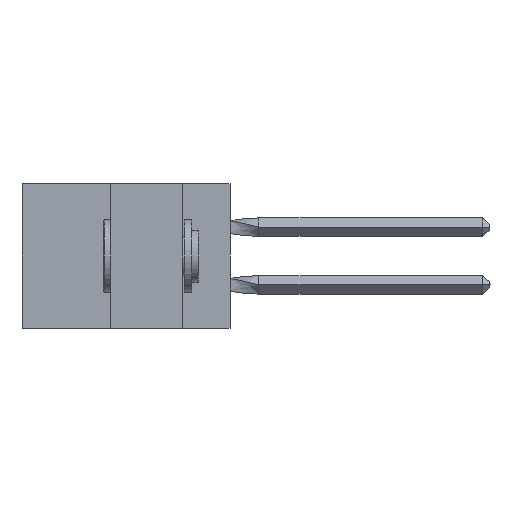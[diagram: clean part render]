
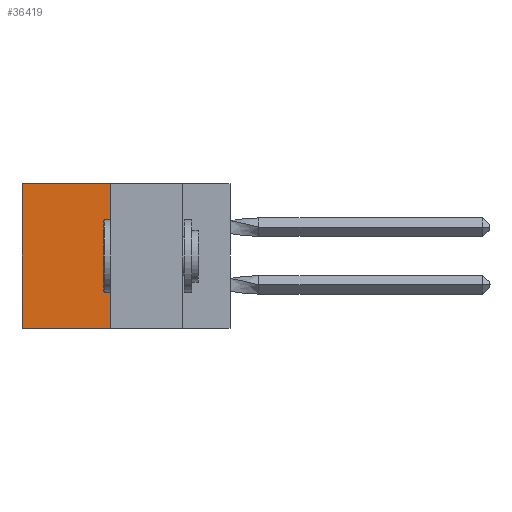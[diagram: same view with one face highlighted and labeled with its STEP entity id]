
A CAD part, left-side view. The second image highlights one B-rep face of the part: STEP entity #36419.
In plain terms, the highlighted planar face has unit normal (-1, 0, 0).
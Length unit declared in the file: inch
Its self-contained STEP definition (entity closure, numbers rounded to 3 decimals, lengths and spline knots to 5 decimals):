
#1017 = PLANE ( 'NONE',  #31629 ) ;
#3175 = ORIENTED_EDGE ( 'NONE', *, *, #29544, .T. ) ;
#3420 = CARTESIAN_POINT ( 'NONE',  ( 0.305, 0.72, -0.5 ) ) ;
#3736 = DIRECTION ( 'NONE',  ( 0., 1., 0. ) ) ;
#3953 = DIRECTION ( 'NONE',  ( 0., 1., 0. ) ) ;
#4171 = CARTESIAN_POINT ( 'NONE',  ( 0.305, 0.413, -0.5 ) ) ;
#5881 = DIRECTION ( 'NONE',  ( 0., 0., -1. ) ) ;
#6220 = EDGE_CURVE ( 'NONE', #6625, #37331, #10451, .T. ) ;
#6625 = VERTEX_POINT ( 'NONE', #23867 ) ;
#7702 = VECTOR ( 'NONE', #5881, 39.37008 ) ;
#7864 = EDGE_LOOP ( 'NONE', ( #3175, #37650, #36208, #18212 ) ) ;
#9058 = VECTOR ( 'NONE', #36589, 39.37008 ) ;
#10451 = LINE ( 'NONE', #34421, #17787 ) ;
#15440 = CARTESIAN_POINT ( 'NONE',  ( 0.305, 0.413, -0.5 ) ) ;
#16715 = DIRECTION ( 'NONE',  ( 0., 0., -1. ) ) ;
#16761 = CARTESIAN_POINT ( 'NONE',  ( 0.305, 0.72, 0. ) ) ;
#17018 = VERTEX_POINT ( 'NONE', #3420 ) ;
#17787 = VECTOR ( 'NONE', #3736, 39.37008 ) ;
#18212 = ORIENTED_EDGE ( 'NONE', *, *, #6220, .T. ) ;
#21100 = CARTESIAN_POINT ( 'NONE',  ( 0.305, 0.413, -0.5 ) ) ;
#22587 = CARTESIAN_POINT ( 'NONE',  ( 0.305, 0.413, -0.5 ) ) ;
#22821 = LINE ( 'NONE', #22587, #34063 ) ;
#23867 = CARTESIAN_POINT ( 'NONE',  ( 0.305, 0.413, 0. ) ) ;
#24811 = VERTEX_POINT ( 'NONE', #21100 ) ;
#26243 = DIRECTION ( 'NONE',  ( 1., 0., 0. ) ) ;
#26593 = LINE ( 'NONE', #26936, #9058 ) ;
#26936 = CARTESIAN_POINT ( 'NONE',  ( 0.305, 0.72, -0.5 ) ) ;
#28273 = EDGE_CURVE ( 'NONE', #6625, #24811, #31125, .T. ) ;
#29544 = EDGE_CURVE ( 'NONE', #37331, #17018, #26593, .T. ) ;
#31125 = LINE ( 'NONE', #15440, #7702 ) ;
#31296 = EDGE_CURVE ( 'NONE', #24811, #17018, #22821, .T. ) ;
#31629 = AXIS2_PLACEMENT_3D ( 'NONE', #4171, #26243, #16715 ) ;
#34063 = VECTOR ( 'NONE', #3953, 39.37008 ) ;
#34421 = CARTESIAN_POINT ( 'NONE',  ( 0.305, 0.413, 0. ) ) ;
#35328 = FACE_OUTER_BOUND ( 'NONE', #7864, .T. ) ;
#36208 = ORIENTED_EDGE ( 'NONE', *, *, #28273, .F. ) ;
#36419 = ADVANCED_FACE ( 'NONE', ( #35328 ), #1017, .F. ) ;
#36589 = DIRECTION ( 'NONE',  ( 0., 0., -1. ) ) ;
#37331 = VERTEX_POINT ( 'NONE', #16761 ) ;
#37650 = ORIENTED_EDGE ( 'NONE', *, *, #31296, .F. ) ;
